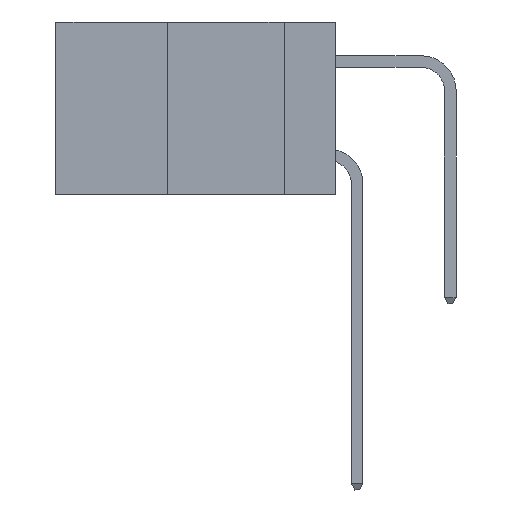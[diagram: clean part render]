
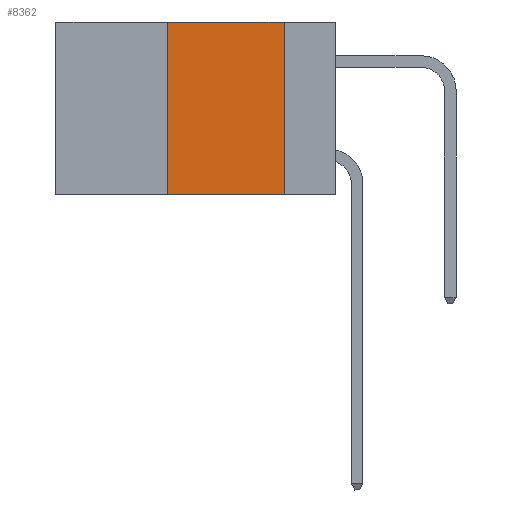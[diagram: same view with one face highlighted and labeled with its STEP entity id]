
A CAD part, left-side view. The second image highlights one B-rep face of the part: STEP entity #8362.
In plain terms, the highlighted planar face has unit normal (-1, 0, 0).
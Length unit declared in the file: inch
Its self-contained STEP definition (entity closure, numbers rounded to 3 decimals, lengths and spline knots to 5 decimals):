
#31 = ORIENTED_EDGE ( 'NONE', *, *, #10252, .F. ) ;
#131 = DIRECTION ( 'NONE',  ( 0., 0., -1. ) ) ;
#262 = VERTEX_POINT ( 'NONE', #13910 ) ;
#504 = CARTESIAN_POINT ( 'NONE',  ( 0., 0.11, 0. ) ) ;
#2260 = CARTESIAN_POINT ( 'NONE',  ( 0., 0.36, -0.37 ) ) ;
#2526 = AXIS2_PLACEMENT_3D ( 'NONE', #8707, #8887, #131 ) ;
#3894 = CARTESIAN_POINT ( 'NONE',  ( 0., 0.11, 0. ) ) ;
#4387 = DIRECTION ( 'NONE',  ( 0., -1., 0. ) ) ;
#4469 = VECTOR ( 'NONE', #4387, 39.37008 ) ;
#4629 = LINE ( 'NONE', #3894, #11794 ) ;
#5046 = VERTEX_POINT ( 'NONE', #504 ) ;
#5084 = ORIENTED_EDGE ( 'NONE', *, *, #10342, .F. ) ;
#5631 = LINE ( 'NONE', #8649, #4469 ) ;
#5731 = LINE ( 'NONE', #14303, #16235 ) ;
#5999 = VECTOR ( 'NONE', #16705, 39.37008 ) ;
#6657 = CARTESIAN_POINT ( 'NONE',  ( 0., 0.36, 0. ) ) ;
#6724 = VERTEX_POINT ( 'NONE', #2260 ) ;
#7106 = ORIENTED_EDGE ( 'NONE', *, *, #12168, .T. ) ;
#7863 = ORIENTED_EDGE ( 'NONE', *, *, #18241, .F. ) ;
#8362 = ADVANCED_FACE ( 'NONE', ( #10754 ), #11446, .F. ) ;
#8649 = CARTESIAN_POINT ( 'NONE',  ( 0., 0.6, 0. ) ) ;
#8707 = CARTESIAN_POINT ( 'NONE',  ( 0., 0.6, 0. ) ) ;
#8887 = DIRECTION ( 'NONE',  ( 1., 0., 0. ) ) ;
#10252 = EDGE_CURVE ( 'NONE', #6724, #11976, #17380, .T. ) ;
#10342 = EDGE_CURVE ( 'NONE', #5046, #262, #4629, .T. ) ;
#10491 = EDGE_LOOP ( 'NONE', ( #5084, #7863, #31, #7106 ) ) ;
#10754 = FACE_OUTER_BOUND ( 'NONE', #10491, .T. ) ;
#11446 = PLANE ( 'NONE',  #2526 ) ;
#11794 = VECTOR ( 'NONE', #13888, 39.37008 ) ;
#11976 = VERTEX_POINT ( 'NONE', #15507 ) ;
#12168 = EDGE_CURVE ( 'NONE', #6724, #262, #5731, .T. ) ;
#13888 = DIRECTION ( 'NONE',  ( 0., 0., -1. ) ) ;
#13910 = CARTESIAN_POINT ( 'NONE',  ( 0., 0.11, -0.37 ) ) ;
#14122 = DIRECTION ( 'NONE',  ( 0., -1., 0. ) ) ;
#14303 = CARTESIAN_POINT ( 'NONE',  ( 0., 0.6, -0.37 ) ) ;
#15507 = CARTESIAN_POINT ( 'NONE',  ( 0., 0.36, 0. ) ) ;
#16235 = VECTOR ( 'NONE', #14122, 39.37008 ) ;
#16705 = DIRECTION ( 'NONE',  ( 0., 0., 1. ) ) ;
#17380 = LINE ( 'NONE', #6657, #5999 ) ;
#18241 = EDGE_CURVE ( 'NONE', #11976, #5046, #5631, .T. ) ;
